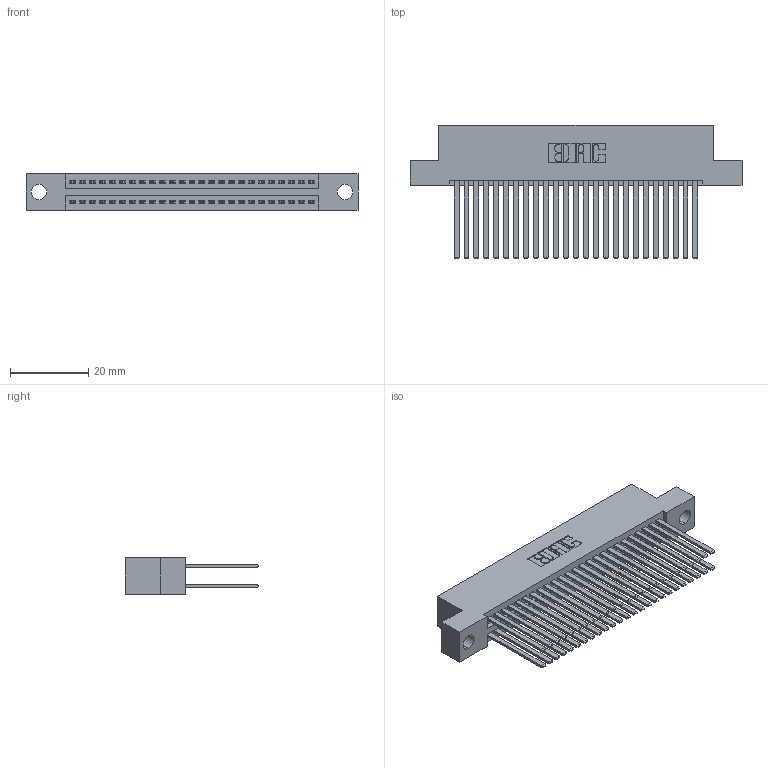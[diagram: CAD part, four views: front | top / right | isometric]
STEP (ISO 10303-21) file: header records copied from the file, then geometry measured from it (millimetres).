
FILE_DESCRIPTION (( 'STEP AP203' ), '1' );
FILE_NAME ('395-050-544-204.STEP', '2018-11-20T09:15:44', ( '' ), ( '' ), 'SwSTEP 2.0', 'SolidWorks 2016', '' );
FILE_SCHEMA (( 'CONFIG_CONTROL_DESIGN' ));
Length unit declared in the file: inch
Products named in the file (3): 345-292-001_345-293-144; 395-050-544-204; 345 Part_Flush Mounting Lugs - 0.156 Dia-TH
Assembly tree (51 placements, depth 2):
  395-050-544-204
    345 Part_Flush Mounting Lugs - 0.156 Dia-TH
    345-292-001_345-293-144  x50
Bounding box: 84.71 x 33.96 x 9.4 mm (x, y, z)
Volume: 8684 mm3; surface area: 14376.6 mm2
Topology: 51 solids, 51 shells, 2326 faces, 6891 edges, 4526 vertices
Faces by surface type: plane 1530, cylinder 796
Entity records: 21723 total; most frequent: CARTESIAN_POINT 3656, ORIENTED_EDGE 3590, DIRECTION 3243, EDGE_CURVE 1795, LINE 1567, VECTOR 1567, VERTEX_POINT 1194, AXIS2_PLACEMENT_3D 838
